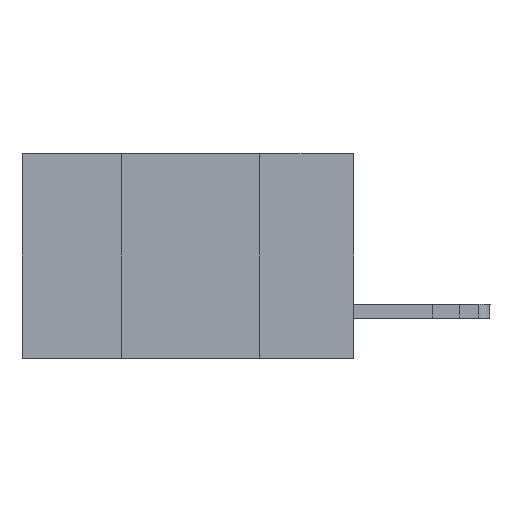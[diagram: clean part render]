
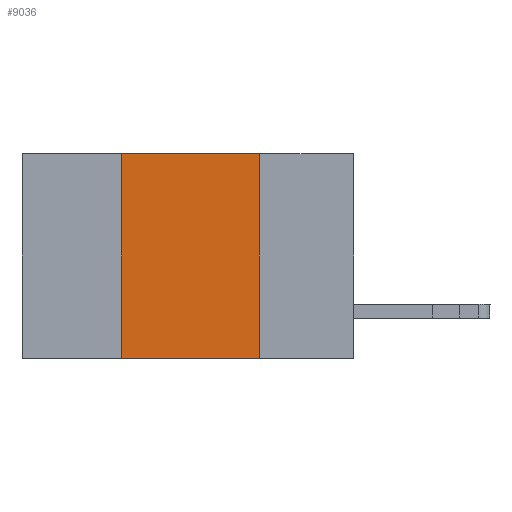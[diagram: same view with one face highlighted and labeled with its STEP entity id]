
A CAD part, left-side view. The second image highlights one B-rep face of the part: STEP entity #9036.
In plain terms, the highlighted planar face has unit normal (-1, 0, 0).
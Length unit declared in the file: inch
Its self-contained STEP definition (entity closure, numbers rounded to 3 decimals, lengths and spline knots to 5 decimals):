
#972 = CARTESIAN_POINT ( 'NONE',  ( 0., 0.6, 0. ) ) ;
#1515 = EDGE_CURVE ( 'NONE', #11279, #30275, #5422, .T. ) ;
#1878 = ORIENTED_EDGE ( 'NONE', *, *, #13313, .F. ) ;
#2094 = PLANE ( 'NONE',  #6809 ) ;
#4539 = FACE_OUTER_BOUND ( 'NONE', #19050, .T. ) ;
#4655 = VECTOR ( 'NONE', #27120, 39.37008 ) ;
#5277 = DIRECTION ( 'NONE',  ( 0., 0., -1. ) ) ;
#5422 = LINE ( 'NONE', #17412, #6007 ) ;
#6007 = VECTOR ( 'NONE', #5277, 39.37008 ) ;
#6684 = DIRECTION ( 'NONE',  ( 1., 0., 0. ) ) ;
#6809 = AXIS2_PLACEMENT_3D ( 'NONE', #13587, #6684, #15769 ) ;
#7690 = CARTESIAN_POINT ( 'NONE',  ( 0., 0.6, -0.37 ) ) ;
#9036 = ADVANCED_FACE ( 'NONE', ( #4539 ), #2094, .F. ) ;
#9537 = CARTESIAN_POINT ( 'NONE',  ( 0., 0.42, 0. ) ) ;
#9698 = DIRECTION ( 'NONE',  ( 0., 0., 1. ) ) ;
#11279 = VERTEX_POINT ( 'NONE', #20738 ) ;
#11364 = VECTOR ( 'NONE', #9698, 39.37008 ) ;
#11816 = EDGE_CURVE ( 'NONE', #13161, #18538, #23589, .T. ) ;
#11979 = CARTESIAN_POINT ( 'NONE',  ( 0., 0.17, -0.37 ) ) ;
#12017 = VECTOR ( 'NONE', #24509, 39.37008 ) ;
#13161 = VERTEX_POINT ( 'NONE', #26068 ) ;
#13313 = EDGE_CURVE ( 'NONE', #18538, #11279, #24661, .T. ) ;
#13587 = CARTESIAN_POINT ( 'NONE',  ( 0., 0.6, 0. ) ) ;
#15274 = ORIENTED_EDGE ( 'NONE', *, *, #11816, .F. ) ;
#15769 = DIRECTION ( 'NONE',  ( 0., 0., -1. ) ) ;
#17412 = CARTESIAN_POINT ( 'NONE',  ( 0., 0.17, 0. ) ) ;
#18538 = VERTEX_POINT ( 'NONE', #22888 ) ;
#19050 = EDGE_LOOP ( 'NONE', ( #22310, #1878, #15274, #29150 ) ) ;
#19176 = EDGE_CURVE ( 'NONE', #13161, #30275, #19882, .T. ) ;
#19882 = LINE ( 'NONE', #7690, #12017 ) ;
#20738 = CARTESIAN_POINT ( 'NONE',  ( 0., 0.17, 0. ) ) ;
#22310 = ORIENTED_EDGE ( 'NONE', *, *, #1515, .F. ) ;
#22888 = CARTESIAN_POINT ( 'NONE',  ( 0., 0.42, 0. ) ) ;
#23589 = LINE ( 'NONE', #9537, #11364 ) ;
#24509 = DIRECTION ( 'NONE',  ( 0., -1., 0. ) ) ;
#24661 = LINE ( 'NONE', #972, #4655 ) ;
#26068 = CARTESIAN_POINT ( 'NONE',  ( 0., 0.42, -0.37 ) ) ;
#27120 = DIRECTION ( 'NONE',  ( 0., -1., 0. ) ) ;
#29150 = ORIENTED_EDGE ( 'NONE', *, *, #19176, .T. ) ;
#30275 = VERTEX_POINT ( 'NONE', #11979 ) ;
